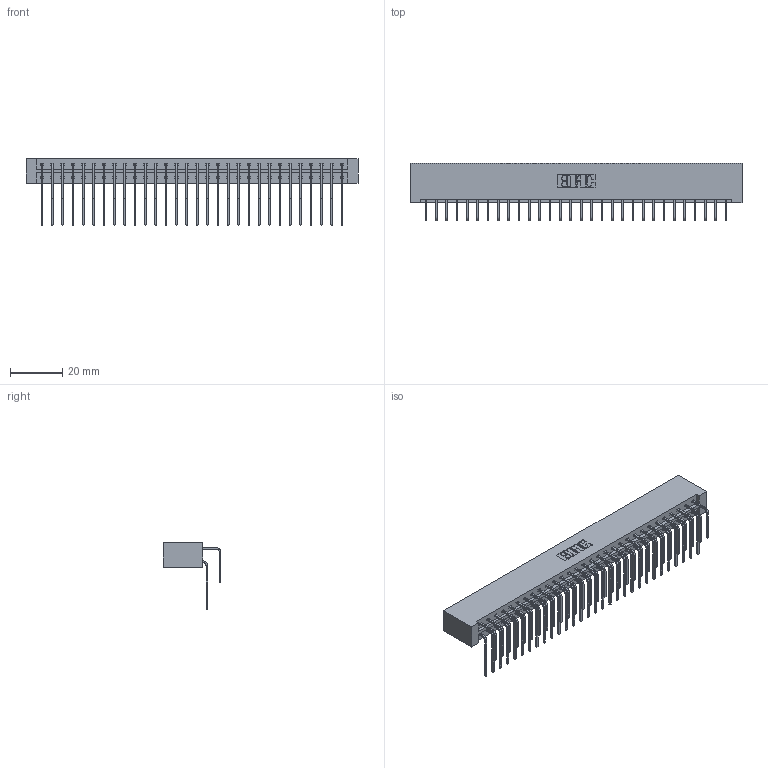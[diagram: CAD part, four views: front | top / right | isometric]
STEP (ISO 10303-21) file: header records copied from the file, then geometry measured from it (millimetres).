
FILE_DESCRIPTION (( 'STEP AP203' ), '1' );
FILE_NAME ('833-060-558-201.STEP', '2020-06-05T04:37:16', ( '' ), ( '' ), 'SwSTEP 2.0', 'SolidWorks 2020', '' );
FILE_SCHEMA (( 'CONFIG_CONTROL_DESIGN' ));
Length unit declared in the file: inch
Products named in the file (4): 345-292-001_558 Tail - 2; 833 Part_Lugless; 833-060-558-201; 345-292-001_558 559 Tail - 1
Assembly tree (61 placements, depth 2):
  833-060-558-201
    833 Part_Lugless
    345-292-001_558 559 Tail - 1  x30
    345-292-001_558 Tail - 2  x30
Bounding box: 127.13 x 22.17 x 25.53 mm (x, y, z)
Volume: 13845.1 mm3; surface area: 17987.8 mm2
Topology: 61 solids, 61 shells, 3346 faces, 9947 edges, 6550 vertices
Faces by surface type: plane 2346, cylinder 1000
Entity records: 22359 total; most frequent: CARTESIAN_POINT 3769, ORIENTED_EDGE 3654, DIRECTION 3215, EDGE_CURVE 1827, LINE 1667, VECTOR 1667, VERTEX_POINT 1214, AXIS2_PLACEMENT_3D 774
